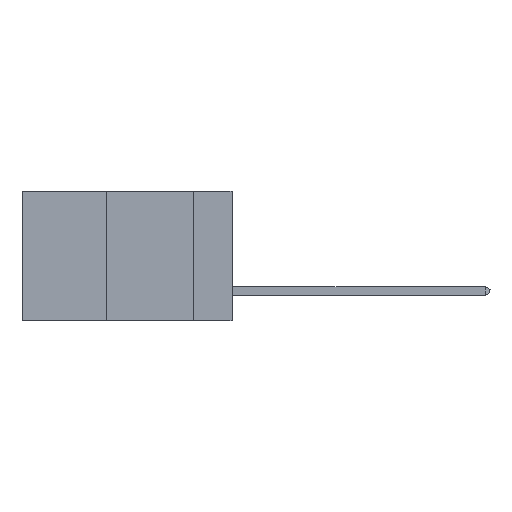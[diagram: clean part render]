
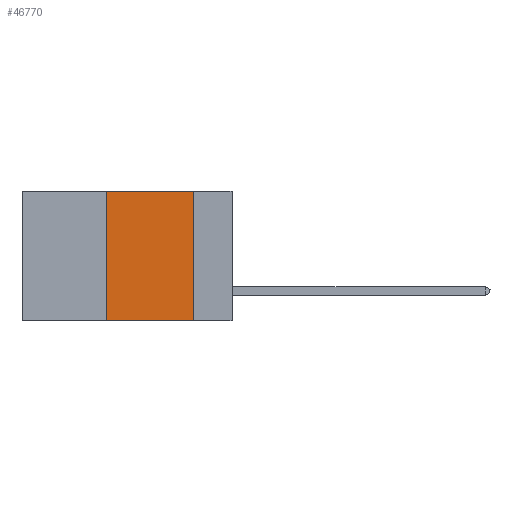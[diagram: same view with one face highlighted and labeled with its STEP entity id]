
A CAD part, left-side view. The second image highlights one B-rep face of the part: STEP entity #46770.
In plain terms, the highlighted planar face has unit normal (-1, 0, 0).
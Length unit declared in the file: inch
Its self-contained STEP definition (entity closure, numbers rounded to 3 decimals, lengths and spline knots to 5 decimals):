
#939 = ORIENTED_EDGE ( 'NONE', *, *, #27346, .T. ) ;
#1011 = VERTEX_POINT ( 'NONE', #25251 ) ;
#1821 = LINE ( 'NONE', #14442, #40356 ) ;
#3157 = DIRECTION ( 'NONE',  ( 0., 0., -1. ) ) ;
#5136 = DIRECTION ( 'NONE',  ( 0., 0., 1. ) ) ;
#6991 = VERTEX_POINT ( 'NONE', #46689 ) ;
#7064 = CARTESIAN_POINT ( 'NONE',  ( 0., 0.6, 0. ) ) ;
#8919 = AXIS2_PLACEMENT_3D ( 'NONE', #7064, #33150, #36938 ) ;
#13648 = EDGE_LOOP ( 'NONE', ( #16651, #20551, #24532, #939 ) ) ;
#14442 = CARTESIAN_POINT ( 'NONE',  ( 0., 0.11, 0. ) ) ;
#15041 = DIRECTION ( 'NONE',  ( 0., -1., 0. ) ) ;
#15403 = CARTESIAN_POINT ( 'NONE',  ( 0., 0.11, 0. ) ) ;
#15568 = CARTESIAN_POINT ( 'NONE',  ( 0., 0.36, 0. ) ) ;
#16010 = VECTOR ( 'NONE', #15041, 39.37008 ) ;
#16651 = ORIENTED_EDGE ( 'NONE', *, *, #33679, .F. ) ;
#20551 = ORIENTED_EDGE ( 'NONE', *, *, #43294, .F. ) ;
#20656 = VERTEX_POINT ( 'NONE', #25843 ) ;
#23021 = VERTEX_POINT ( 'NONE', #15403 ) ;
#23586 = DIRECTION ( 'NONE',  ( 0., -1., 0. ) ) ;
#24532 = ORIENTED_EDGE ( 'NONE', *, *, #25998, .F. ) ;
#25251 = CARTESIAN_POINT ( 'NONE',  ( 0., 0.36, 0. ) ) ;
#25843 = CARTESIAN_POINT ( 'NONE',  ( 0., 0.11, -0.37 ) ) ;
#25998 = EDGE_CURVE ( 'NONE', #6991, #1011, #43510, .T. ) ;
#27346 = EDGE_CURVE ( 'NONE', #6991, #20656, #28547, .T. ) ;
#28547 = LINE ( 'NONE', #45977, #40737 ) ;
#31368 = FACE_OUTER_BOUND ( 'NONE', #13648, .T. ) ;
#33150 = DIRECTION ( 'NONE',  ( 1., 0., 0. ) ) ;
#33679 = EDGE_CURVE ( 'NONE', #23021, #20656, #1821, .T. ) ;
#36938 = DIRECTION ( 'NONE',  ( 0., 0., -1. ) ) ;
#37560 = CARTESIAN_POINT ( 'NONE',  ( 0., 0.6, 0. ) ) ;
#40356 = VECTOR ( 'NONE', #3157, 39.37008 ) ;
#40661 = PLANE ( 'NONE',  #8919 ) ;
#40737 = VECTOR ( 'NONE', #23586, 39.37008 ) ;
#42323 = VECTOR ( 'NONE', #5136, 39.37008 ) ;
#43294 = EDGE_CURVE ( 'NONE', #1011, #23021, #45784, .T. ) ;
#43510 = LINE ( 'NONE', #15568, #42323 ) ;
#45784 = LINE ( 'NONE', #37560, #16010 ) ;
#45977 = CARTESIAN_POINT ( 'NONE',  ( 0., 0.6, -0.37 ) ) ;
#46689 = CARTESIAN_POINT ( 'NONE',  ( 0., 0.36, -0.37 ) ) ;
#46770 = ADVANCED_FACE ( 'NONE', ( #31368 ), #40661, .F. ) ;
